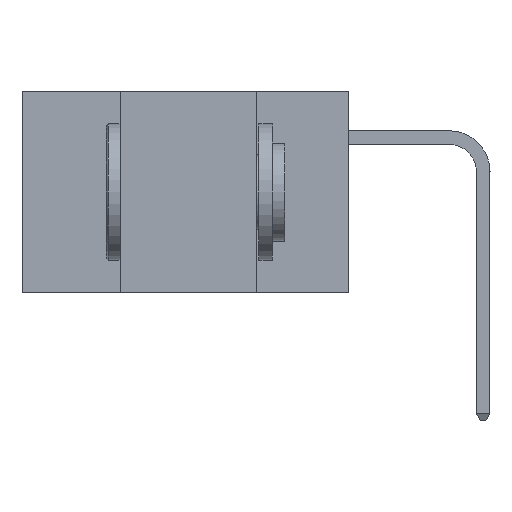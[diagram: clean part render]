
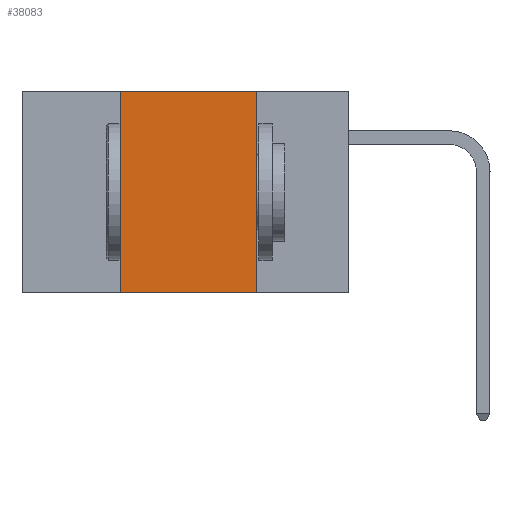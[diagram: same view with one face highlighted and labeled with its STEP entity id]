
A CAD part, left-side view. The second image highlights one B-rep face of the part: STEP entity #38083.
In plain terms, the highlighted planar face has unit normal (-1, 0, 0).
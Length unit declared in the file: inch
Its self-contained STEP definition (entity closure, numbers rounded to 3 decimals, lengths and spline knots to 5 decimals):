
#363 = CARTESIAN_POINT ( 'NONE',  ( 0., 0.17, 0. ) ) ;
#622 = ORIENTED_EDGE ( 'NONE', *, *, #36979, .F. ) ;
#1233 = LINE ( 'NONE', #363, #17092 ) ;
#1718 = CARTESIAN_POINT ( 'NONE',  ( 0., 0.6, -0.37 ) ) ;
#2381 = ORIENTED_EDGE ( 'NONE', *, *, #14008, .F. ) ;
#3598 = DIRECTION ( 'NONE',  ( 0., 0., -1. ) ) ;
#5430 = PLANE ( 'NONE',  #28970 ) ;
#6290 = VERTEX_POINT ( 'NONE', #8613 ) ;
#6531 = FACE_OUTER_BOUND ( 'NONE', #22037, .T. ) ;
#7017 = LINE ( 'NONE', #1718, #36929 ) ;
#8613 = CARTESIAN_POINT ( 'NONE',  ( 0., 0.42, 0. ) ) ;
#9243 = ORIENTED_EDGE ( 'NONE', *, *, #24113, .T. ) ;
#11793 = CARTESIAN_POINT ( 'NONE',  ( 0., 0.6, 0. ) ) ;
#13235 = CARTESIAN_POINT ( 'NONE',  ( 0., 0.6, 0. ) ) ;
#14008 = EDGE_CURVE ( 'NONE', #39118, #6290, #23787, .T. ) ;
#14304 = CARTESIAN_POINT ( 'NONE',  ( 0., 0.17, -0.37 ) ) ;
#15003 = DIRECTION ( 'NONE',  ( 0., 0., -1. ) ) ;
#15123 = ORIENTED_EDGE ( 'NONE', *, *, #19055, .F. ) ;
#15968 = VECTOR ( 'NONE', #16430, 39.37008 ) ;
#16430 = DIRECTION ( 'NONE',  ( 0., -1., 0. ) ) ;
#17092 = VECTOR ( 'NONE', #3598, 39.37008 ) ;
#19055 = EDGE_CURVE ( 'NONE', #6290, #23030, #32912, .T. ) ;
#19944 = CARTESIAN_POINT ( 'NONE',  ( 0., 0.42, -0.37 ) ) ;
#22037 = EDGE_LOOP ( 'NONE', ( #622, #15123, #2381, #9243 ) ) ;
#22791 = VECTOR ( 'NONE', #32921, 39.37008 ) ;
#23030 = VERTEX_POINT ( 'NONE', #40412 ) ;
#23787 = LINE ( 'NONE', #29726, #22791 ) ;
#24113 = EDGE_CURVE ( 'NONE', #39118, #30688, #7017, .T. ) ;
#28970 = AXIS2_PLACEMENT_3D ( 'NONE', #11793, #34065, #15003 ) ;
#29726 = CARTESIAN_POINT ( 'NONE',  ( 0., 0.42, 0. ) ) ;
#30688 = VERTEX_POINT ( 'NONE', #14304 ) ;
#32912 = LINE ( 'NONE', #13235, #15968 ) ;
#32921 = DIRECTION ( 'NONE',  ( 0., 0., 1. ) ) ;
#34065 = DIRECTION ( 'NONE',  ( 1., 0., 0. ) ) ;
#36477 = DIRECTION ( 'NONE',  ( 0., -1., 0. ) ) ;
#36929 = VECTOR ( 'NONE', #36477, 39.37008 ) ;
#36979 = EDGE_CURVE ( 'NONE', #23030, #30688, #1233, .T. ) ;
#38083 = ADVANCED_FACE ( 'NONE', ( #6531 ), #5430, .F. ) ;
#39118 = VERTEX_POINT ( 'NONE', #19944 ) ;
#40412 = CARTESIAN_POINT ( 'NONE',  ( 0., 0.17, 0. ) ) ;
